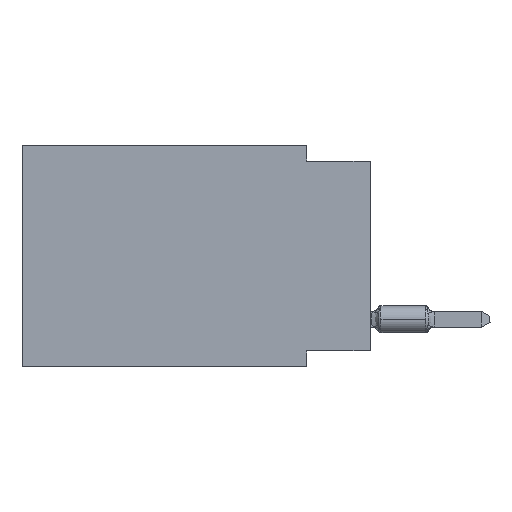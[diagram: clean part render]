
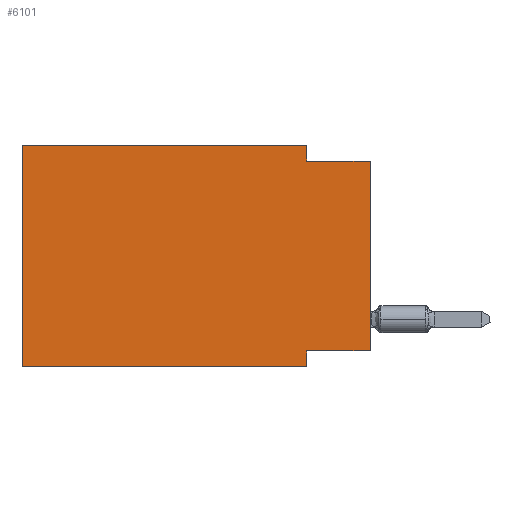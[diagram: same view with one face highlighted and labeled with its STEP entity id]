
A CAD part, left-side view. The second image highlights one B-rep face of the part: STEP entity #6101.
In plain terms, the highlighted planar face has unit normal (-1, 0, 0).
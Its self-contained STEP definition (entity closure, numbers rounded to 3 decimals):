
#1 = VERTEX_POINT ( 'NONE', #16767 ) ;
#649 = LINE ( 'NONE', #2159, #11742 ) ;
#1010 = LINE ( 'NONE', #4690, #22359 ) ;
#1469 = ORIENTED_EDGE ( 'NONE', *, *, #11393, .F. ) ;
#1882 = DIRECTION ( 'NONE',  ( 0., 0., -1. ) ) ;
#2159 = CARTESIAN_POINT ( 'NONE',  ( 0., 13.97, -8.89 ) ) ;
#2510 = VERTEX_POINT ( 'NONE', #14804 ) ;
#3239 = VECTOR ( 'NONE', #20000, 1000. ) ;
#3328 = VECTOR ( 'NONE', #8617, 1000. ) ;
#3352 = VECTOR ( 'NONE', #11731, 1000. ) ;
#3933 = VECTOR ( 'NONE', #22574, 1000. ) ;
#3987 = CARTESIAN_POINT ( 'NONE',  ( 0., 13.97, 0. ) ) ;
#4296 = CARTESIAN_POINT ( 'NONE',  ( 0., 2.54, 0. ) ) ;
#4690 = CARTESIAN_POINT ( 'NONE',  ( 0., 0., 0. ) ) ;
#4863 = CARTESIAN_POINT ( 'NONE',  ( 0., 2.54, -8.255 ) ) ;
#4970 = LINE ( 'NONE', #15511, #3328 ) ;
#5405 = AXIS2_PLACEMENT_3D ( 'NONE', #17451, #19292, #13881 ) ;
#5509 = FACE_OUTER_BOUND ( 'NONE', #10573, .T. ) ;
#5911 = CARTESIAN_POINT ( 'NONE',  ( 0., 0., -8.255 ) ) ;
#6101 = ADVANCED_FACE ( 'NONE', ( #5509 ), #20904, .F. ) ;
#7530 = CARTESIAN_POINT ( 'NONE',  ( 0., 0., -0.635 ) ) ;
#7665 = DIRECTION ( 'NONE',  ( 0., -1., 0. ) ) ;
#7723 = EDGE_CURVE ( 'NONE', #1, #14529, #14696, .T. ) ;
#8074 = ORIENTED_EDGE ( 'NONE', *, *, #16069, .T. ) ;
#8427 = LINE ( 'NONE', #17618, #10829 ) ;
#8617 = DIRECTION ( 'NONE',  ( 0., -1., 0. ) ) ;
#8870 = ORIENTED_EDGE ( 'NONE', *, *, #19908, .T. ) ;
#9971 = VERTEX_POINT ( 'NONE', #4863 ) ;
#10188 = CARTESIAN_POINT ( 'NONE',  ( 0., 2.54, -8.89 ) ) ;
#10290 = CARTESIAN_POINT ( 'NONE',  ( 0., 0., -8.255 ) ) ;
#10301 = LINE ( 'NONE', #17308, #13251 ) ;
#10573 = EDGE_LOOP ( 'NONE', ( #8074, #13685, #1469, #16823, #14528, #8870, #10702, #16556 ) ) ;
#10702 = ORIENTED_EDGE ( 'NONE', *, *, #17386, .F. ) ;
#10829 = VECTOR ( 'NONE', #1882, 1000. ) ;
#11146 = DIRECTION ( 'NONE',  ( 0., -1., 0. ) ) ;
#11393 = EDGE_CURVE ( 'NONE', #13318, #2510, #8427, .T. ) ;
#11463 = DIRECTION ( 'NONE',  ( 0., 0., 1. ) ) ;
#11731 = DIRECTION ( 'NONE',  ( 0., 0., -1. ) ) ;
#11742 = VECTOR ( 'NONE', #7665, 1000. ) ;
#13047 = EDGE_CURVE ( 'NONE', #18310, #9971, #15565, .T. ) ;
#13122 = VERTEX_POINT ( 'NONE', #7530 ) ;
#13251 = VECTOR ( 'NONE', #11146, 1000. ) ;
#13318 = VERTEX_POINT ( 'NONE', #4296 ) ;
#13685 = ORIENTED_EDGE ( 'NONE', *, *, #19130, .F. ) ;
#13881 = DIRECTION ( 'NONE',  ( 0., 0., -1. ) ) ;
#14528 = ORIENTED_EDGE ( 'NONE', *, *, #7723, .F. ) ;
#14529 = VERTEX_POINT ( 'NONE', #3987 ) ;
#14696 = LINE ( 'NONE', #18266, #3239 ) ;
#14804 = CARTESIAN_POINT ( 'NONE',  ( 0., 2.54, -0.635 ) ) ;
#15281 = CARTESIAN_POINT ( 'NONE',  ( 0., 2.54, -8.89 ) ) ;
#15511 = CARTESIAN_POINT ( 'NONE',  ( 0., 0., -0.635 ) ) ;
#15565 = LINE ( 'NONE', #10290, #3933 ) ;
#16069 = EDGE_CURVE ( 'NONE', #18310, #13122, #1010, .T. ) ;
#16556 = ORIENTED_EDGE ( 'NONE', *, *, #13047, .F. ) ;
#16767 = CARTESIAN_POINT ( 'NONE',  ( 0., 13.97, -8.89 ) ) ;
#16823 = ORIENTED_EDGE ( 'NONE', *, *, #21338, .F. ) ;
#17308 = CARTESIAN_POINT ( 'NONE',  ( 0., 13.97, 0. ) ) ;
#17386 = EDGE_CURVE ( 'NONE', #9971, #21253, #22293, .T. ) ;
#17451 = CARTESIAN_POINT ( 'NONE',  ( 0., 13.97, 0. ) ) ;
#17618 = CARTESIAN_POINT ( 'NONE',  ( 0., 2.54, 0. ) ) ;
#18266 = CARTESIAN_POINT ( 'NONE',  ( 0., 13.97, 0. ) ) ;
#18310 = VERTEX_POINT ( 'NONE', #5911 ) ;
#19130 = EDGE_CURVE ( 'NONE', #2510, #13122, #4970, .T. ) ;
#19292 = DIRECTION ( 'NONE',  ( 1., 0., 0. ) ) ;
#19908 = EDGE_CURVE ( 'NONE', #1, #21253, #649, .T. ) ;
#20000 = DIRECTION ( 'NONE',  ( 0., 0., 1. ) ) ;
#20904 = PLANE ( 'NONE',  #5405 ) ;
#21253 = VERTEX_POINT ( 'NONE', #10188 ) ;
#21338 = EDGE_CURVE ( 'NONE', #14529, #13318, #10301, .T. ) ;
#22293 = LINE ( 'NONE', #15281, #3352 ) ;
#22359 = VECTOR ( 'NONE', #11463, 1000. ) ;
#22574 = DIRECTION ( 'NONE',  ( 0., 1., 0. ) ) ;
